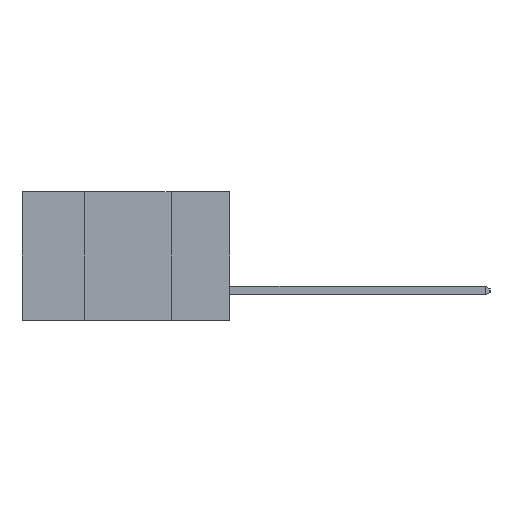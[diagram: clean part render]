
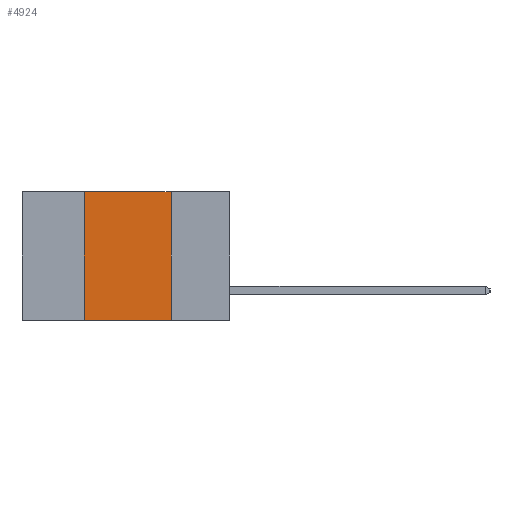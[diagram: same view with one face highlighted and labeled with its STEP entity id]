
A CAD part, left-side view. The second image highlights one B-rep face of the part: STEP entity #4924.
In plain terms, the highlighted planar face has unit normal (-1, 0, 0).
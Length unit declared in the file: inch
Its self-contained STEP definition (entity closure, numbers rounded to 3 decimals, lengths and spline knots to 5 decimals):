
#23 = PLANE ( 'NONE',  #4671 ) ;
#90 = CARTESIAN_POINT ( 'NONE',  ( 0., 0.6, 0. ) ) ;
#313 = LINE ( 'NONE', #5461, #5494 ) ;
#536 = EDGE_LOOP ( 'NONE', ( #11383, #3861, #870, #8176 ) ) ;
#870 = ORIENTED_EDGE ( 'NONE', *, *, #7608, .F. ) ;
#1666 = LINE ( 'NONE', #10315, #6695 ) ;
#3129 = VECTOR ( 'NONE', #8315, 39.37008 ) ;
#3861 = ORIENTED_EDGE ( 'NONE', *, *, #5141, .F. ) ;
#4191 = DIRECTION ( 'NONE',  ( 1., 0., 0. ) ) ;
#4671 = AXIS2_PLACEMENT_3D ( 'NONE', #90, #4191, #12625 ) ;
#4924 = ADVANCED_FACE ( 'NONE', ( #8159 ), #23, .F. ) ;
#5141 = EDGE_CURVE ( 'NONE', #10020, #8172, #12713, .T. ) ;
#5149 = VECTOR ( 'NONE', #9637, 39.37008 ) ;
#5461 = CARTESIAN_POINT ( 'NONE',  ( 0., 0.17, 0. ) ) ;
#5494 = VECTOR ( 'NONE', #10209, 39.37008 ) ;
#5524 = VERTEX_POINT ( 'NONE', #10218 ) ;
#5525 = EDGE_CURVE ( 'NONE', #5524, #11538, #7681, .T. ) ;
#5564 = DIRECTION ( 'NONE',  ( 0., 0., 1. ) ) ;
#5824 = CARTESIAN_POINT ( 'NONE',  ( 0., 0.6, 0. ) ) ;
#6695 = VECTOR ( 'NONE', #5564, 39.37008 ) ;
#7238 = CARTESIAN_POINT ( 'NONE',  ( 0., 0.17, 0. ) ) ;
#7608 = EDGE_CURVE ( 'NONE', #5524, #10020, #1666, .T. ) ;
#7681 = LINE ( 'NONE', #11531, #5149 ) ;
#8159 = FACE_OUTER_BOUND ( 'NONE', #536, .T. ) ;
#8172 = VERTEX_POINT ( 'NONE', #7238 ) ;
#8176 = ORIENTED_EDGE ( 'NONE', *, *, #5525, .T. ) ;
#8258 = EDGE_CURVE ( 'NONE', #8172, #11538, #313, .T. ) ;
#8315 = DIRECTION ( 'NONE',  ( 0., -1., 0. ) ) ;
#9637 = DIRECTION ( 'NONE',  ( 0., -1., 0. ) ) ;
#10020 = VERTEX_POINT ( 'NONE', #10143 ) ;
#10143 = CARTESIAN_POINT ( 'NONE',  ( 0., 0.42, 0. ) ) ;
#10209 = DIRECTION ( 'NONE',  ( 0., 0., -1. ) ) ;
#10218 = CARTESIAN_POINT ( 'NONE',  ( 0., 0.42, -0.37 ) ) ;
#10315 = CARTESIAN_POINT ( 'NONE',  ( 0., 0.42, 0. ) ) ;
#10633 = CARTESIAN_POINT ( 'NONE',  ( 0., 0.17, -0.37 ) ) ;
#11383 = ORIENTED_EDGE ( 'NONE', *, *, #8258, .F. ) ;
#11531 = CARTESIAN_POINT ( 'NONE',  ( 0., 0.6, -0.37 ) ) ;
#11538 = VERTEX_POINT ( 'NONE', #10633 ) ;
#12625 = DIRECTION ( 'NONE',  ( 0., 0., -1. ) ) ;
#12713 = LINE ( 'NONE', #5824, #3129 ) ;
